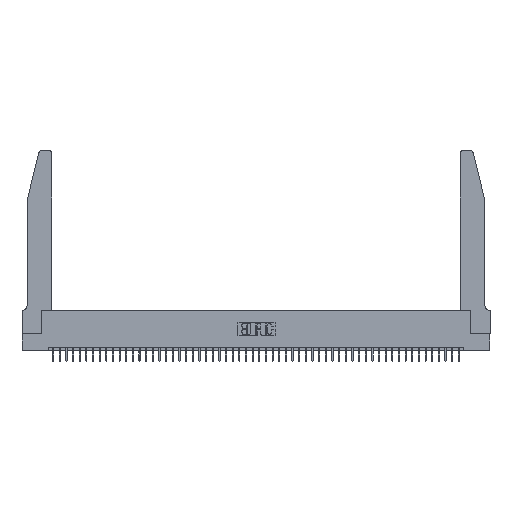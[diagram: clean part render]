
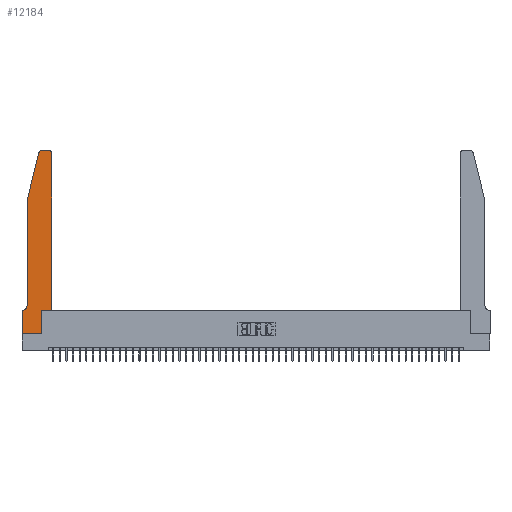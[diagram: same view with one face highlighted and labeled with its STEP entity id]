
A CAD part, top view. The second image highlights one B-rep face of the part: STEP entity #12184.
In plain terms, the highlighted planar face has unit normal (0, 0, 1).
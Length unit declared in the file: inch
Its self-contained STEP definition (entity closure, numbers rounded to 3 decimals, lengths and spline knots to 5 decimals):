
#77 = VERTEX_POINT ( 'NONE', #44229 ) ;
#117 = CARTESIAN_POINT ( 'NONE',  ( 0.4505, 0.35, 0.37 ) ) ;
#1157 = VERTEX_POINT ( 'NONE', #23681 ) ;
#1482 = VECTOR ( 'NONE', #34637, 39.37008 ) ;
#2552 = CARTESIAN_POINT ( 'NONE',  ( 0.0755, 2., 0.37 ) ) ;
#2607 = DIRECTION ( 'NONE',  ( 0., 1., 0. ) ) ;
#3038 = EDGE_CURVE ( 'NONE', #33415, #7209, #33524, .T. ) ;
#3745 = ORIENTED_EDGE ( 'NONE', *, *, #48321, .T. ) ;
#3885 = ORIENTED_EDGE ( 'NONE', *, *, #32971, .T. ) ;
#4156 = EDGE_CURVE ( 'NONE', #10902, #47094, #18656, .T. ) ;
#4804 = LINE ( 'NONE', #38221, #6058 ) ;
#4853 = DIRECTION ( 'NONE',  ( 0., 0., 1. ) ) ;
#6058 = VECTOR ( 'NONE', #30656, 39.37008 ) ;
#6296 = CARTESIAN_POINT ( 'NONE',  ( 0.4505, 0.35, 0.37 ) ) ;
#6693 = VERTEX_POINT ( 'NONE', #6296 ) ;
#7044 = CIRCLE ( 'NONE', #30502, 0.03 ) ;
#7209 = VERTEX_POINT ( 'NONE', #36437 ) ;
#7438 = DIRECTION ( 'NONE',  ( 0., 0., 1. ) ) ;
#8474 = CARTESIAN_POINT ( 'NONE',  ( 0.284, 2.72, 0.37 ) ) ;
#9426 = ORIENTED_EDGE ( 'NONE', *, *, #31541, .T. ) ;
#10329 = VECTOR ( 'NONE', #14882, 39.37008 ) ;
#10387 = DIRECTION ( 'NONE',  ( 0., -1., 0. ) ) ;
#10902 = VERTEX_POINT ( 'NONE', #18993 ) ;
#10985 = ORIENTED_EDGE ( 'NONE', *, *, #4156, .T. ) ;
#12184 = ADVANCED_FACE ( 'NONE', ( #40506 ), #47009, .T. ) ;
#14882 = DIRECTION ( 'NONE',  ( -1., 0., 0. ) ) ;
#15093 = CARTESIAN_POINT ( 'NONE',  ( 0., 0.35, 0.37 ) ) ;
#15153 = VERTEX_POINT ( 'NONE', #37728 ) ;
#15214 = EDGE_CURVE ( 'NONE', #47094, #15153, #46615, .T. ) ;
#15463 = LINE ( 'NONE', #25987, #42498 ) ;
#16050 = LINE ( 'NONE', #41797, #43695 ) ;
#16121 = EDGE_LOOP ( 'NONE', ( #46469, #3885, #10985, #45125, #9426, #49886, #45825, #20021, #45075, #3745, #43331, #40392 ) ) ;
#18222 = AXIS2_PLACEMENT_3D ( 'NONE', #32385, #4853, #33273 ) ;
#18656 = LINE ( 'NONE', #22094, #39484 ) ;
#18993 = CARTESIAN_POINT ( 'NONE',  ( 0.25487, 2.72718, 0.37 ) ) ;
#19467 = CARTESIAN_POINT ( 'NONE',  ( 0.0055, 0.42, 0.37 ) ) ;
#19622 = DIRECTION ( 'NONE',  ( -1., 0., 0. ) ) ;
#20021 = ORIENTED_EDGE ( 'NONE', *, *, #41799, .T. ) ;
#22094 = CARTESIAN_POINT ( 'NONE',  ( 0.0755, 2., 0.37 ) ) ;
#23459 = DIRECTION ( 'NONE',  ( 1., 0., 0. ) ) ;
#23489 = CARTESIAN_POINT ( 'NONE',  ( 0., 0.35, 0.37 ) ) ;
#23666 = AXIS2_PLACEMENT_3D ( 'NONE', #23489, #7438, #50272 ) ;
#23681 = CARTESIAN_POINT ( 'NONE',  ( 0.4205, 2.75, 0.37 ) ) ;
#25578 = AXIS2_PLACEMENT_3D ( 'NONE', #19467, #42457, #19622 ) ;
#25987 = CARTESIAN_POINT ( 'NONE',  ( 0., 0., 0.37 ) ) ;
#27408 = CARTESIAN_POINT ( 'NONE',  ( 0.0755, 0.35, 0.37 ) ) ;
#28176 = EDGE_CURVE ( 'NONE', #38930, #1157, #49377, .T. ) ;
#28376 = CARTESIAN_POINT ( 'NONE',  ( 0.4505, 2.72, 0.37 ) ) ;
#30217 = VERTEX_POINT ( 'NONE', #35511 ) ;
#30257 = DIRECTION ( 'NONE',  ( -0.239, -0.971, 0. ) ) ;
#30502 = AXIS2_PLACEMENT_3D ( 'NONE', #8474, #36045, #48261 ) ;
#30656 = DIRECTION ( 'NONE',  ( 0., 1., 0. ) ) ;
#31541 = EDGE_CURVE ( 'NONE', #15153, #77, #36608, .T. ) ;
#32385 = CARTESIAN_POINT ( 'NONE',  ( 0.4205, 2.72, 0.37 ) ) ;
#32971 = EDGE_CURVE ( 'NONE', #30217, #10902, #7044, .T. ) ;
#32991 = VERTEX_POINT ( 'NONE', #48425 ) ;
#33183 = CARTESIAN_POINT ( 'NONE',  ( 0.0755, 2., 0.37 ) ) ;
#33273 = DIRECTION ( 'NONE',  ( 1., 0., 0. ) ) ;
#33344 = EDGE_CURVE ( 'NONE', #77, #33415, #45070, .T. ) ;
#33415 = VERTEX_POINT ( 'NONE', #15093 ) ;
#33524 = LINE ( 'NONE', #44056, #34749 ) ;
#34009 = EDGE_CURVE ( 'NONE', #6693, #38930, #16050, .T. ) ;
#34442 = CARTESIAN_POINT ( 'NONE',  ( 0.2605, 2.75, 0.37 ) ) ;
#34637 = DIRECTION ( 'NONE',  ( -1., 0., 0. ) ) ;
#34749 = VECTOR ( 'NONE', #44401, 39.37008 ) ;
#35511 = CARTESIAN_POINT ( 'NONE',  ( 0.284, 2.75, 0.37 ) ) ;
#36045 = DIRECTION ( 'NONE',  ( 0., 0., 1. ) ) ;
#36093 = LINE ( 'NONE', #34442, #10329 ) ;
#36437 = CARTESIAN_POINT ( 'NONE',  ( 0., 0., 0.37 ) ) ;
#36608 = CIRCLE ( 'NONE', #25578, 0.07 ) ;
#36831 = CARTESIAN_POINT ( 'NONE',  ( 0.2865, 0.35, 0.37 ) ) ;
#37491 = DIRECTION ( 'NONE',  ( 1., 0., 0. ) ) ;
#37539 = EDGE_CURVE ( 'NONE', #1157, #30217, #36093, .T. ) ;
#37728 = CARTESIAN_POINT ( 'NONE',  ( 0.0755, 0.42, 0.37 ) ) ;
#37814 = VECTOR ( 'NONE', #23459, 39.37008 ) ;
#38221 = CARTESIAN_POINT ( 'NONE',  ( 0.2865, 0.35, 0.37 ) ) ;
#38930 = VERTEX_POINT ( 'NONE', #28376 ) ;
#39484 = VECTOR ( 'NONE', #30257, 39.37008 ) ;
#40392 = ORIENTED_EDGE ( 'NONE', *, *, #28176, .T. ) ;
#40506 = FACE_OUTER_BOUND ( 'NONE', #16121, .T. ) ;
#41797 = CARTESIAN_POINT ( 'NONE',  ( 0.4505, 0.35, 0.37 ) ) ;
#41799 = EDGE_CURVE ( 'NONE', #7209, #32991, #15463, .T. ) ;
#42457 = DIRECTION ( 'NONE',  ( 0., 0., -1. ) ) ;
#42498 = VECTOR ( 'NONE', #37491, 39.37008 ) ;
#42525 = VERTEX_POINT ( 'NONE', #36831 ) ;
#43331 = ORIENTED_EDGE ( 'NONE', *, *, #34009, .T. ) ;
#43695 = VECTOR ( 'NONE', #2607, 39.37008 ) ;
#44056 = CARTESIAN_POINT ( 'NONE',  ( 0., 0., 0.37 ) ) ;
#44229 = CARTESIAN_POINT ( 'NONE',  ( 0.0055, 0.35, 0.37 ) ) ;
#44401 = DIRECTION ( 'NONE',  ( 0., -1., 0. ) ) ;
#45070 = LINE ( 'NONE', #27408, #1482 ) ;
#45075 = ORIENTED_EDGE ( 'NONE', *, *, #45684, .T. ) ;
#45125 = ORIENTED_EDGE ( 'NONE', *, *, #15214, .T. ) ;
#45684 = EDGE_CURVE ( 'NONE', #32991, #42525, #4804, .T. ) ;
#45825 = ORIENTED_EDGE ( 'NONE', *, *, #3038, .T. ) ;
#46469 = ORIENTED_EDGE ( 'NONE', *, *, #37539, .T. ) ;
#46615 = LINE ( 'NONE', #2552, #49670 ) ;
#47009 = PLANE ( 'NONE',  #23666 ) ;
#47094 = VERTEX_POINT ( 'NONE', #33183 ) ;
#48261 = DIRECTION ( 'NONE',  ( 1., 0., 0. ) ) ;
#48270 = LINE ( 'NONE', #117, #37814 ) ;
#48321 = EDGE_CURVE ( 'NONE', #42525, #6693, #48270, .T. ) ;
#48425 = CARTESIAN_POINT ( 'NONE',  ( 0.2865, 0., 0.37 ) ) ;
#49377 = CIRCLE ( 'NONE', #18222, 0.03 ) ;
#49670 = VECTOR ( 'NONE', #10387, 39.37008 ) ;
#49886 = ORIENTED_EDGE ( 'NONE', *, *, #33344, .T. ) ;
#50272 = DIRECTION ( 'NONE',  ( 1., 0., 0. ) ) ;
